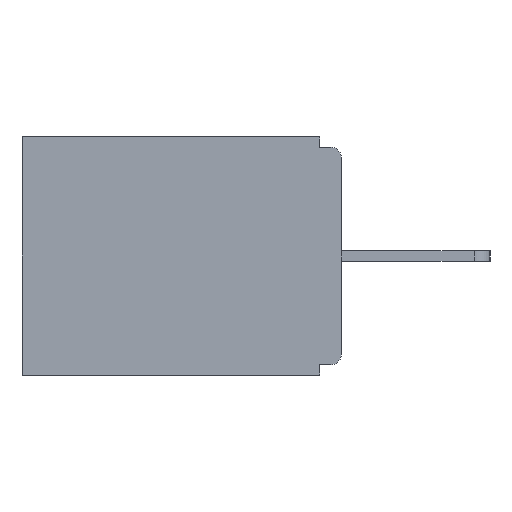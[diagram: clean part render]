
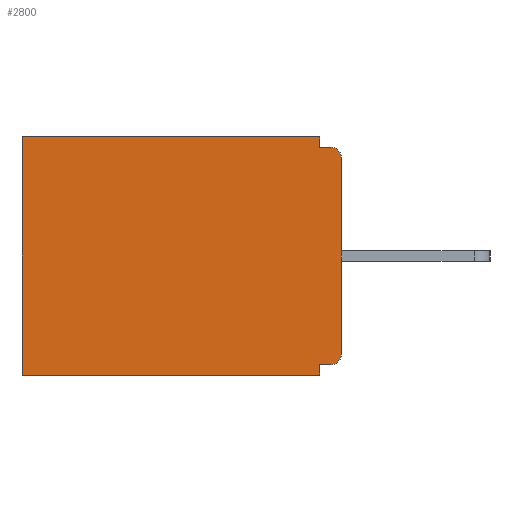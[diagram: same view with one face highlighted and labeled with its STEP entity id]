
A CAD part, left-side view. The second image highlights one B-rep face of the part: STEP entity #2800.
In plain terms, the highlighted planar face has unit normal (-1, 0, 0).
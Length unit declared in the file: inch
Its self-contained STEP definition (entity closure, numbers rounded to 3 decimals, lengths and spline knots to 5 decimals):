
#13 = DIRECTION ( 'NONE',  ( 0., 1., 0. ) ) ;
#166 = DIRECTION ( 'NONE',  ( -1., 0., 0. ) ) ;
#250 = EDGE_LOOP ( 'NONE', ( #12143, #18921, #24368, #3147, #6044, #6793, #2678, #21132, #25318, #10704 ) ) ;
#394 = LINE ( 'NONE', #16794, #1764 ) ;
#790 = DIRECTION ( 'NONE',  ( 0., 1., 0. ) ) ;
#1662 = CARTESIAN_POINT ( 'NONE',  ( 0.298, 0., 0. ) ) ;
#1720 = VERTEX_POINT ( 'NONE', #16748 ) ;
#1764 = VECTOR ( 'NONE', #25058, 39.37008 ) ;
#1827 = CARTESIAN_POINT ( 'NONE',  ( 0.298, 0.015, -0.03 ) ) ;
#1839 = CARTESIAN_POINT ( 'NONE',  ( 0.298, 0.46, 0. ) ) ;
#2631 = CARTESIAN_POINT ( 'NONE',  ( 0.298, 0., -0.313 ) ) ;
#2678 = ORIENTED_EDGE ( 'NONE', *, *, #9733, .F. ) ;
#2800 = ADVANCED_FACE ( 'NONE', ( #10224 ), #16444, .F. ) ;
#3147 = ORIENTED_EDGE ( 'NONE', *, *, #12738, .T. ) ;
#4124 = LINE ( 'NONE', #14421, #8627 ) ;
#4541 = VERTEX_POINT ( 'NONE', #21123 ) ;
#4613 = CIRCLE ( 'NONE', #17230, 0.015 ) ;
#5982 = CARTESIAN_POINT ( 'NONE',  ( 0.298, 0.015, -0.313 ) ) ;
#6044 = ORIENTED_EDGE ( 'NONE', *, *, #18933, .T. ) ;
#6793 = ORIENTED_EDGE ( 'NONE', *, *, #8197, .F. ) ;
#8014 = VERTEX_POINT ( 'NONE', #24403 ) ;
#8197 = EDGE_CURVE ( 'NONE', #4541, #23846, #394, .T. ) ;
#8454 = DIRECTION ( 'NONE',  ( 0., 0., -1. ) ) ;
#8627 = VECTOR ( 'NONE', #14547, 39.37008 ) ;
#8872 = DIRECTION ( 'NONE',  ( 0., 0., -1. ) ) ;
#9127 = CARTESIAN_POINT ( 'NONE',  ( 0.298, 0., 0. ) ) ;
#9733 = EDGE_CURVE ( 'NONE', #1720, #4541, #23981, .T. ) ;
#10224 = FACE_OUTER_BOUND ( 'NONE', #250, .T. ) ;
#10623 = VECTOR ( 'NONE', #12324, 39.37008 ) ;
#10704 = ORIENTED_EDGE ( 'NONE', *, *, #15816, .F. ) ;
#10948 = DIRECTION ( 'NONE',  ( -1., 0., 0. ) ) ;
#11011 = DIRECTION ( 'NONE',  ( 1., 0., 0. ) ) ;
#11248 = CARTESIAN_POINT ( 'NONE',  ( 0.298, 0.46, 0. ) ) ;
#11672 = CIRCLE ( 'NONE', #19455, 0.015 ) ;
#11969 = VECTOR ( 'NONE', #790, 39.37008 ) ;
#12143 = ORIENTED_EDGE ( 'NONE', *, *, #24444, .T. ) ;
#12148 = LINE ( 'NONE', #1839, #14209 ) ;
#12231 = EDGE_CURVE ( 'NONE', #19751, #24840, #15804, .T. ) ;
#12324 = DIRECTION ( 'NONE',  ( 0., -1., 0. ) ) ;
#12550 = DIRECTION ( 'NONE',  ( 0., 0., -1. ) ) ;
#12713 = CARTESIAN_POINT ( 'NONE',  ( 0.298, 0.031, -0.015 ) ) ;
#12738 = EDGE_CURVE ( 'NONE', #14568, #23623, #16284, .T. ) ;
#12853 = VERTEX_POINT ( 'NONE', #20507 ) ;
#13117 = DIRECTION ( 'NONE',  ( 0., 0., -1. ) ) ;
#13415 = EDGE_CURVE ( 'NONE', #8014, #1720, #15674, .T. ) ;
#14088 = CARTESIAN_POINT ( 'NONE',  ( 0.298, 0.031, -0.343 ) ) ;
#14209 = VECTOR ( 'NONE', #12550, 39.37008 ) ;
#14421 = CARTESIAN_POINT ( 'NONE',  ( 0.298, 0.031, -0.343 ) ) ;
#14547 = DIRECTION ( 'NONE',  ( 0., 0., -1. ) ) ;
#14568 = VERTEX_POINT ( 'NONE', #15226 ) ;
#14833 = CARTESIAN_POINT ( 'NONE',  ( 0.298, 0., 0. ) ) ;
#15226 = CARTESIAN_POINT ( 'NONE',  ( 0.298, 0.031, 0. ) ) ;
#15306 = EDGE_CURVE ( 'NONE', #8014, #21592, #4613, .T. ) ;
#15418 = CARTESIAN_POINT ( 'NONE',  ( 0.298, 0., -0.328 ) ) ;
#15674 = LINE ( 'NONE', #15418, #11969 ) ;
#15804 = LINE ( 'NONE', #22610, #10623 ) ;
#15816 = EDGE_CURVE ( 'NONE', #12853, #21592, #20693, .T. ) ;
#16231 = VECTOR ( 'NONE', #13, 39.37008 ) ;
#16284 = LINE ( 'NONE', #1662, #16231 ) ;
#16444 = PLANE ( 'NONE',  #19072 ) ;
#16748 = CARTESIAN_POINT ( 'NONE',  ( 0.298, 0.031, -0.328 ) ) ;
#16794 = CARTESIAN_POINT ( 'NONE',  ( 0.298, 0., -0.343 ) ) ;
#17230 = AXIS2_PLACEMENT_3D ( 'NONE', #5982, #10948, #13117 ) ;
#18598 = CARTESIAN_POINT ( 'NONE',  ( 0.298, 0.015, -0.015 ) ) ;
#18921 = ORIENTED_EDGE ( 'NONE', *, *, #12231, .F. ) ;
#18933 = EDGE_CURVE ( 'NONE', #23623, #23846, #12148, .T. ) ;
#19072 = AXIS2_PLACEMENT_3D ( 'NONE', #9127, #11011, #23340 ) ;
#19455 = AXIS2_PLACEMENT_3D ( 'NONE', #1827, #166, #8454 ) ;
#19751 = VERTEX_POINT ( 'NONE', #12713 ) ;
#20293 = EDGE_CURVE ( 'NONE', #14568, #19751, #4124, .T. ) ;
#20507 = CARTESIAN_POINT ( 'NONE',  ( 0.298, 0., -0.03 ) ) ;
#20693 = LINE ( 'NONE', #14833, #22826 ) ;
#21123 = CARTESIAN_POINT ( 'NONE',  ( 0.298, 0.031, -0.343 ) ) ;
#21132 = ORIENTED_EDGE ( 'NONE', *, *, #13415, .F. ) ;
#21592 = VERTEX_POINT ( 'NONE', #2631 ) ;
#22214 = CARTESIAN_POINT ( 'NONE',  ( 0.298, 0.46, -0.343 ) ) ;
#22610 = CARTESIAN_POINT ( 'NONE',  ( 0.298, 0., -0.015 ) ) ;
#22826 = VECTOR ( 'NONE', #8872, 39.37008 ) ;
#23340 = DIRECTION ( 'NONE',  ( 0., 0., -1. ) ) ;
#23623 = VERTEX_POINT ( 'NONE', #11248 ) ;
#23846 = VERTEX_POINT ( 'NONE', #22214 ) ;
#23981 = LINE ( 'NONE', #14088, #24247 ) ;
#24247 = VECTOR ( 'NONE', #26002, 39.37008 ) ;
#24368 = ORIENTED_EDGE ( 'NONE', *, *, #20293, .F. ) ;
#24403 = CARTESIAN_POINT ( 'NONE',  ( 0.298, 0.015, -0.328 ) ) ;
#24444 = EDGE_CURVE ( 'NONE', #12853, #24840, #11672, .T. ) ;
#24840 = VERTEX_POINT ( 'NONE', #18598 ) ;
#25058 = DIRECTION ( 'NONE',  ( 0., 1., 0. ) ) ;
#25318 = ORIENTED_EDGE ( 'NONE', *, *, #15306, .T. ) ;
#26002 = DIRECTION ( 'NONE',  ( 0., 0., -1. ) ) ;
